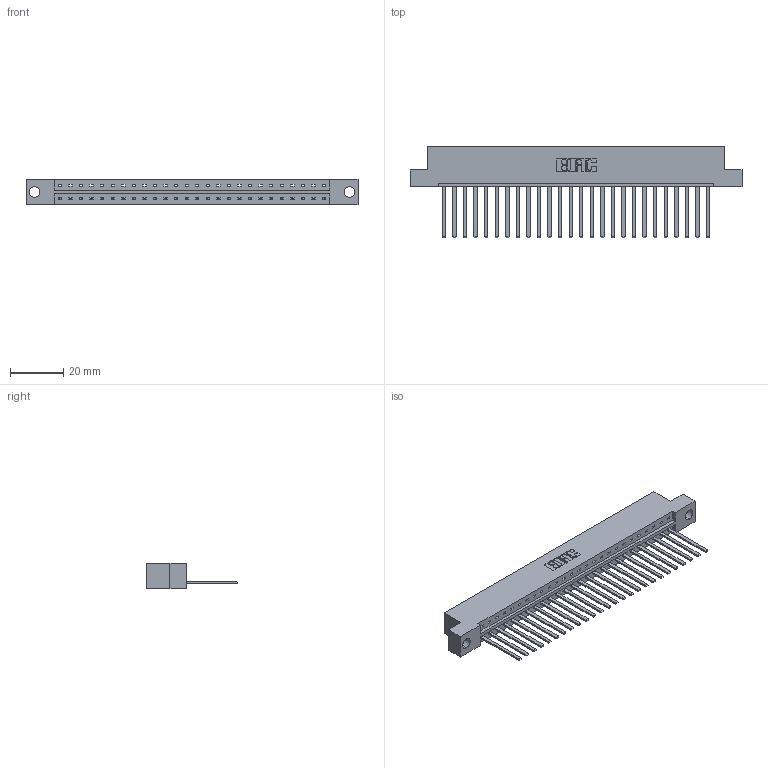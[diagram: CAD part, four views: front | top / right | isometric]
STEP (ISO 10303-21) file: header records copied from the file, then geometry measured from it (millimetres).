
FILE_DESCRIPTION (( 'STEP AP203' ), '1' );
FILE_NAME ('333-026-544-104.STEP', '2018-08-02T13:11:33', ( '' ), ( '' ), 'SwSTEP 2.0', 'SolidWorks 2016', '' );
FILE_SCHEMA (( 'CONFIG_CONTROL_DESIGN' ));
Length unit declared in the file: inch
Products named in the file (3): 345-292-001_345-293-144; 333-026-544-104; 333 Part_Flush - .156 Dia - TH
Assembly tree (27 placements, depth 2):
  333-026-544-104
    333 Part_Flush - .156 Dia - TH
    345-292-001_345-293-144  x26
Bounding box: 124.56 x 34.3 x 9.4 mm (x, y, z)
Volume: 12610.1 mm3; surface area: 14313.6 mm2
Topology: 27 solids, 27 shells, 1466 faces, 4419 edges, 2910 vertices
Faces by surface type: plane 1058, cylinder 408
Entity records: 17783 total; most frequent: CARTESIAN_POINT 3076, ORIENTED_EDGE 3038, DIRECTION 2623, EDGE_CURVE 1519, VECTOR 1395, LINE 1395, VERTEX_POINT 1010, AXIS2_PLACEMENT_3D 614
